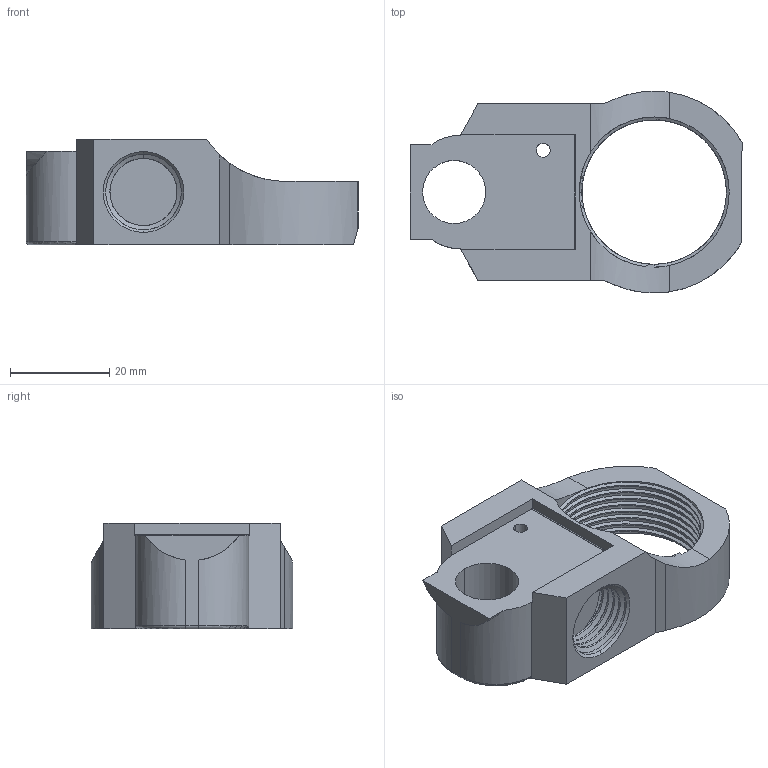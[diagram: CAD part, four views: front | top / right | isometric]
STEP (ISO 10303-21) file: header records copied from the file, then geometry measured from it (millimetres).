
FILE_DESCRIPTION (( 'STEP AP203' ), '1' );
FILE_NAME ('AF-WF-LR-PRT-002-STEP.STEP', '2020-07-21T18:18:57', ( '' ), ( '' ), 'SwSTEP 2.0', 'SolidWorks 2018', '' );
FILE_SCHEMA (( 'CONFIG_CONTROL_DESIGN' ));
Length unit declared in the file: inch
Products named in the file (1): AF-WF-LR-PRT-002-STEP
Bounding box: 66.83 x 40.62 x 21.27 mm (x, y, z)
Volume: 20209 mm3; surface area: 10547.4 mm2
Topology: 1 solids, 1 shells, 110 faces, 304 edges, 195 vertices
Faces by surface type: cylinder 60, plane 22, bspline 14, cone 12, torus 2
Entity records: 8596 total; most frequent: CARTESIAN_POINT 6078, ORIENTED_EDGE 600, DIRECTION 419, EDGE_CURVE 300, VERTEX_POINT 195, AXIS2_PLACEMENT_3D 155, EDGE_LOOP 119, ADVANCED_FACE 110
